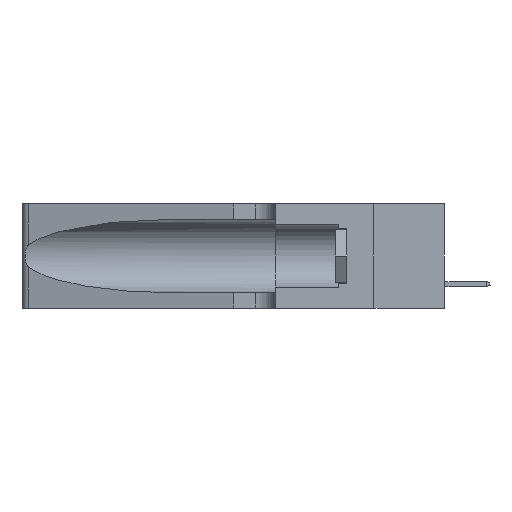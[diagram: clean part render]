
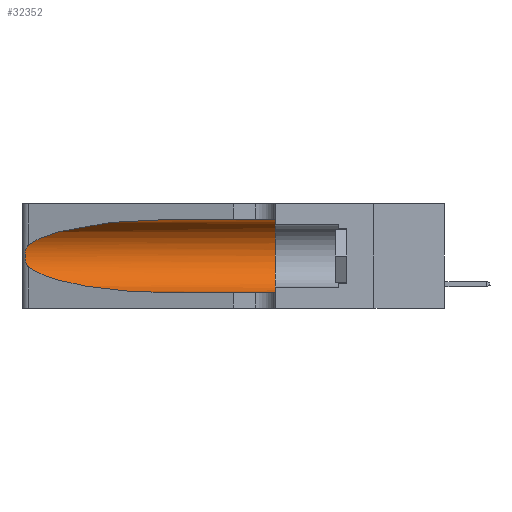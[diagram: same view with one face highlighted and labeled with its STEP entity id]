
A CAD part, left-side view. The second image highlights one B-rep face of the part: STEP entity #32352.
In plain terms, the highlighted cylindrical face has radius 3.308 mm (diameter 6.617 mm), a partial arc.
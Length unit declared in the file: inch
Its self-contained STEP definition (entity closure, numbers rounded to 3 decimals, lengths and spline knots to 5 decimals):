
#288 = CARTESIAN_POINT ( 'NONE',  ( 0.1305, 1.61858, 0.05475 ) ) ;
#329 = ORIENTED_EDGE ( 'NONE', *, *, #4109, .T. ) ;
#1550 = CARTESIAN_POINT ( 'NONE',  ( 0.25555, 1.22994, 0.2215 ) ) ;
#1663 = CARTESIAN_POINT ( 'NONE',  ( 0.25487, 1.22718, 0.22369 ) ) ;
#1778 = CARTESIAN_POINT ( 'NONE',  ( 0.25856, 1.23593, 0.16098 ) ) ;
#1943 = CARTESIAN_POINT ( 'NONE',  ( 0.1305, 1.61858, 0.185 ) ) ;
#2198 = AXIS2_PLACEMENT_3D ( 'NONE', #9750, #32738, #17412 ) ;
#3407 = EDGE_CURVE ( 'NONE', #21198, #29836, #23568, .T. ) ;
#3414 = DIRECTION ( 'NONE',  ( 0., -1., 0. ) ) ;
#3544 = EDGE_CURVE ( 'NONE', #20476, #6699, #7663, .T. ) ;
#3756 = LINE ( 'NONE', #23723, #4972 ) ;
#4007 = ORIENTED_EDGE ( 'NONE', *, *, #20485, .F. ) ;
#4109 = EDGE_CURVE ( 'NONE', #25881, #21198, #17679, .T. ) ;
#4243 = CARTESIAN_POINT ( 'NONE',  ( 0.25854, 1.2359, 0.20912 ) ) ;
#4384 = CARTESIAN_POINT ( 'NONE',  ( 0.18966, 0.96281, 0.05475 ) ) ;
#4525 = DIRECTION ( 'NONE',  ( 0., -1., 0. ) ) ;
#4531 = CARTESIAN_POINT ( 'NONE',  ( 0.2373, 1.15595, 0.28018 ) ) ;
#4972 = VECTOR ( 'NONE', #3414, 39.37008 ) ;
#6502 = CARTESIAN_POINT ( 'NONE',  ( 0.26018, 1.23835, 0.19895 ) ) ;
#6699 = VERTEX_POINT ( 'NONE', #14998 ) ;
#6794 = CARTESIAN_POINT ( 'NONE',  ( 0.18966, 0.96281, 0.31525 ) ) ;
#7663 = CIRCLE ( 'NONE', #2198, 0.13025 ) ;
#8817 = VERTEX_POINT ( 'NONE', #29504 ) ;
#9171 = CARTESIAN_POINT ( 'NONE',  ( 0.25487, 1.22718, 0.14631 ) ) ;
#9275 = CARTESIAN_POINT ( 'NONE',  ( 0.25639, 1.23186, 0.15144 ) ) ;
#9750 = CARTESIAN_POINT ( 'NONE',  ( 0.1305, 0.35, 0.185 ) ) ;
#10458 = AXIS2_PLACEMENT_3D ( 'NONE', #1943, #4525, #24842 ) ;
#12292 = CARTESIAN_POINT ( 'NONE',  ( 0.25487, 1.22718, 0.22369 ) ) ;
#14998 = CARTESIAN_POINT ( 'NONE',  ( 0.1305, 0.35, 0.05475 ) ) ;
#16111 = CARTESIAN_POINT ( 'NONE',  ( 0.1305, 0.35, 0.31525 ) ) ;
#16276 = CARTESIAN_POINT ( 'NONE',  ( 0.25487, 1.22718, 0.14631 ) ) ;
#17188 = CARTESIAN_POINT ( 'NONE',  ( 0.26075, 1.23896, 0.19203 ) ) ;
#17412 = DIRECTION ( 'NONE',  ( 0., 0., 1. ) ) ;
#17535 = CARTESIAN_POINT ( 'NONE',  ( 0.25487, 1.22718, 0.22369 ) ) ;
#17679 =( BOUNDED_CURVE ( )  B_SPLINE_CURVE ( 3, ( #22296, #6794, #4531, #12292 ),
 .UNSPECIFIED., .F., .T. ) 
 B_SPLINE_CURVE_WITH_KNOTS ( ( 4, 4 ),
 ( 1.5708, 2.84003 ),
 .UNSPECIFIED. ) 
 CURVE ( )  GEOMETRIC_REPRESENTATION_ITEM ( )  RATIONAL_B_SPLINE_CURVE ( ( 1., 0.87, 0.87, 1. ) ) 
 REPRESENTATION_ITEM ( '' )  );
#19562 = CARTESIAN_POINT ( 'NONE',  ( 0.25555, 1.22993, 0.14849 ) ) ;
#19801 = CARTESIAN_POINT ( 'NONE',  ( 0.25487, 1.22718, 0.14631 ) ) ;
#20476 = VERTEX_POINT ( 'NONE', #16111 ) ;
#20485 = EDGE_CURVE ( 'NONE', #25881, #20476, #3756, .T. ) ;
#20764 = ORIENTED_EDGE ( 'NONE', *, *, #3544, .F. ) ;
#21007 = DIRECTION ( 'NONE',  ( 0., -1., 0. ) ) ;
#21158 = VECTOR ( 'NONE', #21007, 39.37008 ) ;
#21198 = VERTEX_POINT ( 'NONE', #17535 ) ;
#21317 = ORIENTED_EDGE ( 'NONE', *, *, #24895, .T. ) ;
#21576 =( BOUNDED_CURVE ( )  B_SPLINE_CURVE ( 3, ( #19801, #25040, #4384, #22375 ),
 .UNSPECIFIED., .F., .T. ) 
 B_SPLINE_CURVE_WITH_KNOTS ( ( 4, 4 ),
 ( 3.44316, 4.71239 ),
 .UNSPECIFIED. ) 
 CURVE ( )  GEOMETRIC_REPRESENTATION_ITEM ( )  RATIONAL_B_SPLINE_CURVE ( ( 1., 0.87, 0.87, 1. ) ) 
 REPRESENTATION_ITEM ( '' )  );
#22079 = ORIENTED_EDGE ( 'NONE', *, *, #27459, .T. ) ;
#22227 = CARTESIAN_POINT ( 'NONE',  ( 0.26075, 1.23896, 0.178 ) ) ;
#22296 = CARTESIAN_POINT ( 'NONE',  ( 0.1305, 0.72297, 0.31525 ) ) ;
#22375 = CARTESIAN_POINT ( 'NONE',  ( 0.1305, 0.72297, 0.05475 ) ) ;
#23568 = B_SPLINE_CURVE_WITH_KNOTS ( 'NONE', 3,
 ( #1663, #1550, #29625, #27242, #4243, #6502, #17188, #22227, #29731, #1778, #24571, #9275, #19562, #9171 ),
 .UNSPECIFIED., .F., .F.,
 ( 4, 2, 2, 2, 2, 2, 4 ),
 ( 0., 0.00027, 0.00053, 0.00107, 0.0016, 0.00187, 0.00214 ),
 .UNSPECIFIED. ) ;
#23723 = CARTESIAN_POINT ( 'NONE',  ( 0.1305, 1.61858, 0.31525 ) ) ;
#23929 = CYLINDRICAL_SURFACE ( 'NONE', #10458, 0.13025 ) ;
#23965 = LINE ( 'NONE', #288, #21158 ) ;
#24501 = ORIENTED_EDGE ( 'NONE', *, *, #3407, .T. ) ;
#24571 = CARTESIAN_POINT ( 'NONE',  ( 0.25789, 1.23486, 0.15765 ) ) ;
#24842 = DIRECTION ( 'NONE',  ( 0., 0., -1. ) ) ;
#24895 = EDGE_CURVE ( 'NONE', #8817, #6699, #23965, .T. ) ;
#25040 = CARTESIAN_POINT ( 'NONE',  ( 0.2373, 1.15595, 0.08982 ) ) ;
#25881 = VERTEX_POINT ( 'NONE', #31062 ) ;
#26757 = FACE_OUTER_BOUND ( 'NONE', #32523, .T. ) ;
#27242 = CARTESIAN_POINT ( 'NONE',  ( 0.25787, 1.23484, 0.2124 ) ) ;
#27459 = EDGE_CURVE ( 'NONE', #29836, #8817, #21576, .T. ) ;
#29504 = CARTESIAN_POINT ( 'NONE',  ( 0.1305, 0.72297, 0.05475 ) ) ;
#29625 = CARTESIAN_POINT ( 'NONE',  ( 0.25639, 1.23184, 0.21858 ) ) ;
#29731 = CARTESIAN_POINT ( 'NONE',  ( 0.26017, 1.23833, 0.17102 ) ) ;
#29836 = VERTEX_POINT ( 'NONE', #16276 ) ;
#31062 = CARTESIAN_POINT ( 'NONE',  ( 0.1305, 0.72297, 0.31525 ) ) ;
#32352 = ADVANCED_FACE ( 'NONE', ( #26757 ), #23929, .F. ) ;
#32523 = EDGE_LOOP ( 'NONE', ( #329, #24501, #22079, #21317, #20764, #4007 ) ) ;
#32738 = DIRECTION ( 'NONE',  ( 0., 1., 0. ) ) ;
